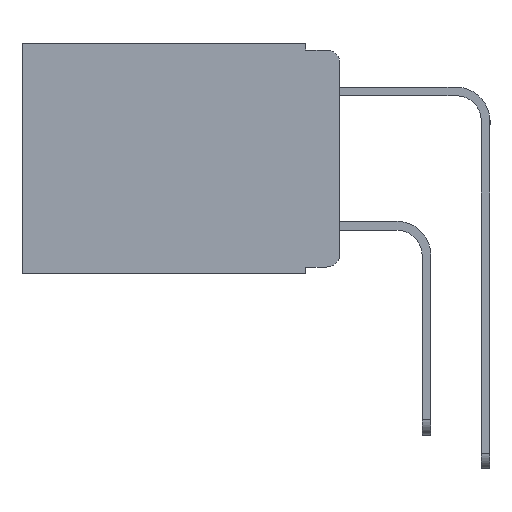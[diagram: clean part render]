
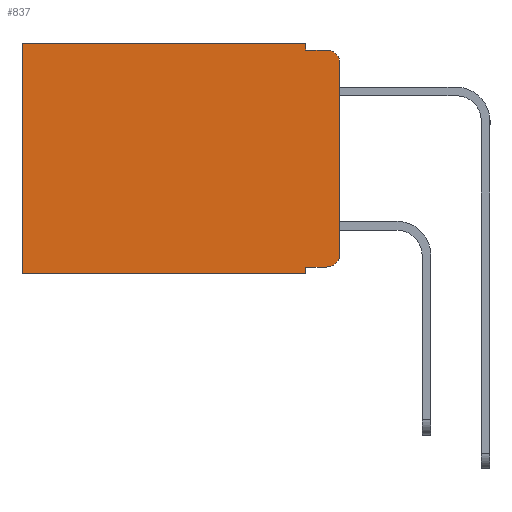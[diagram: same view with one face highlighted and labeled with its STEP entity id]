
A CAD part, left-side view. The second image highlights one B-rep face of the part: STEP entity #837.
In plain terms, the highlighted planar face has unit normal (-1, 0, 0).
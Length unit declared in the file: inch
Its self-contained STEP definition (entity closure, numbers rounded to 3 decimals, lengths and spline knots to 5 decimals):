
#44 = CARTESIAN_POINT ( 'NONE',  ( 0.298, 0., -0.343 ) ) ;
#300 = CIRCLE ( 'NONE', #15026, 0.02 ) ;
#590 = DIRECTION ( 'NONE',  ( 0., 0., -1. ) ) ;
#837 = ADVANCED_FACE ( 'NONE', ( #17397 ), #5609, .F. ) ;
#901 = DIRECTION ( 'NONE',  ( 0., 0., -1. ) ) ;
#1458 = VERTEX_POINT ( 'NONE', #9337 ) ;
#1536 = EDGE_CURVE ( 'NONE', #2580, #4755, #14142, .T. ) ;
#1682 = DIRECTION ( 'NONE',  ( 1., 0., 0. ) ) ;
#1812 = LINE ( 'NONE', #17218, #8643 ) ;
#2066 = CARTESIAN_POINT ( 'NONE',  ( 0.298, 0.473, 0. ) ) ;
#2218 = DIRECTION ( 'NONE',  ( -1., 0., 0. ) ) ;
#2278 = DIRECTION ( 'NONE',  ( 0., -1., 0. ) ) ;
#2351 = VERTEX_POINT ( 'NONE', #14316 ) ;
#2580 = VERTEX_POINT ( 'NONE', #3429 ) ;
#2722 = VECTOR ( 'NONE', #11802, 39.37008 ) ;
#2741 = ORIENTED_EDGE ( 'NONE', *, *, #3618, .F. ) ;
#2819 = CARTESIAN_POINT ( 'NONE',  ( 0.298, 0.051, 0. ) ) ;
#3107 = VECTOR ( 'NONE', #4114, 39.37008 ) ;
#3253 = EDGE_CURVE ( 'NONE', #2351, #4755, #1812, .T. ) ;
#3304 = DIRECTION ( 'NONE',  ( 0., 0., -1. ) ) ;
#3429 = CARTESIAN_POINT ( 'NONE',  ( 0.298, 0.02, -0.333 ) ) ;
#3611 = ORIENTED_EDGE ( 'NONE', *, *, #16328, .F. ) ;
#3618 = EDGE_CURVE ( 'NONE', #8045, #9236, #7158, .T. ) ;
#3931 = VECTOR ( 'NONE', #590, 39.37008 ) ;
#3989 = CARTESIAN_POINT ( 'NONE',  ( 0.298, 0.473, 0. ) ) ;
#4114 = DIRECTION ( 'NONE',  ( 0., 1., 0. ) ) ;
#4152 = AXIS2_PLACEMENT_3D ( 'NONE', #11030, #1682, #10770 ) ;
#4343 = LINE ( 'NONE', #2066, #3931 ) ;
#4755 = VERTEX_POINT ( 'NONE', #6860 ) ;
#4945 = VERTEX_POINT ( 'NONE', #16501 ) ;
#4966 = CARTESIAN_POINT ( 'NONE',  ( 0.298, 0.473, -0.343 ) ) ;
#5494 = ORIENTED_EDGE ( 'NONE', *, *, #7493, .T. ) ;
#5609 = PLANE ( 'NONE',  #4152 ) ;
#5837 = DIRECTION ( 'NONE',  ( -1., 0., 0. ) ) ;
#5928 = ORIENTED_EDGE ( 'NONE', *, *, #15274, .T. ) ;
#6097 = DIRECTION ( 'NONE',  ( 0., 1., 0. ) ) ;
#6785 = ORIENTED_EDGE ( 'NONE', *, *, #3253, .F. ) ;
#6860 = CARTESIAN_POINT ( 'NONE',  ( 0.298, 0., -0.313 ) ) ;
#7158 = LINE ( 'NONE', #44, #3107 ) ;
#7361 = AXIS2_PLACEMENT_3D ( 'NONE', #12222, #5837, #11647 ) ;
#7493 = EDGE_CURVE ( 'NONE', #12480, #13552, #8487, .T. ) ;
#8045 = VERTEX_POINT ( 'NONE', #13812 ) ;
#8256 = EDGE_CURVE ( 'NONE', #2351, #1458, #300, .T. ) ;
#8300 = EDGE_CURVE ( 'NONE', #4945, #2580, #17018, .T. ) ;
#8487 = LINE ( 'NONE', #8618, #15176 ) ;
#8618 = CARTESIAN_POINT ( 'NONE',  ( 0.298, 0., 0. ) ) ;
#8643 = VECTOR ( 'NONE', #17198, 39.37008 ) ;
#8720 = EDGE_CURVE ( 'NONE', #11048, #1458, #13982, .T. ) ;
#9236 = VERTEX_POINT ( 'NONE', #4966 ) ;
#9337 = CARTESIAN_POINT ( 'NONE',  ( 0.298, 0.02, -0.01 ) ) ;
#10429 = VECTOR ( 'NONE', #2278, 39.37008 ) ;
#10770 = DIRECTION ( 'NONE',  ( 0., 0., -1. ) ) ;
#10808 = LINE ( 'NONE', #14158, #16948 ) ;
#10879 = LINE ( 'NONE', #13105, #2722 ) ;
#11030 = CARTESIAN_POINT ( 'NONE',  ( 0.298, 0., 0. ) ) ;
#11048 = VERTEX_POINT ( 'NONE', #15604 ) ;
#11429 = CARTESIAN_POINT ( 'NONE',  ( 0.298, 0.051, -0.01 ) ) ;
#11647 = DIRECTION ( 'NONE',  ( 0., 0., -1. ) ) ;
#11802 = DIRECTION ( 'NONE',  ( 0., 0., -1. ) ) ;
#12164 = ORIENTED_EDGE ( 'NONE', *, *, #8720, .F. ) ;
#12222 = CARTESIAN_POINT ( 'NONE',  ( 0.298, 0.02, -0.313 ) ) ;
#12480 = VERTEX_POINT ( 'NONE', #2819 ) ;
#12805 = EDGE_CURVE ( 'NONE', #12480, #11048, #10879, .T. ) ;
#12919 = CARTESIAN_POINT ( 'NONE',  ( 0.298, 0.02, -0.03 ) ) ;
#13105 = CARTESIAN_POINT ( 'NONE',  ( 0.298, 0.051, 0. ) ) ;
#13552 = VERTEX_POINT ( 'NONE', #3989 ) ;
#13576 = VECTOR ( 'NONE', #15730, 39.37008 ) ;
#13812 = CARTESIAN_POINT ( 'NONE',  ( 0.298, 0.051, -0.343 ) ) ;
#13982 = LINE ( 'NONE', #11429, #10429 ) ;
#14121 = EDGE_LOOP ( 'NONE', ( #6785, #14409, #12164, #15800, #5494, #5928, #2741, #3611, #14423, #16845 ) ) ;
#14142 = CIRCLE ( 'NONE', #7361, 0.02 ) ;
#14158 = CARTESIAN_POINT ( 'NONE',  ( 0.298, 0.051, 0. ) ) ;
#14316 = CARTESIAN_POINT ( 'NONE',  ( 0.298, 0., -0.03 ) ) ;
#14409 = ORIENTED_EDGE ( 'NONE', *, *, #8256, .T. ) ;
#14423 = ORIENTED_EDGE ( 'NONE', *, *, #8300, .T. ) ;
#15026 = AXIS2_PLACEMENT_3D ( 'NONE', #12919, #2218, #901 ) ;
#15176 = VECTOR ( 'NONE', #6097, 39.37008 ) ;
#15274 = EDGE_CURVE ( 'NONE', #13552, #9236, #4343, .T. ) ;
#15604 = CARTESIAN_POINT ( 'NONE',  ( 0.298, 0.051, -0.01 ) ) ;
#15730 = DIRECTION ( 'NONE',  ( 0., -1., 0. ) ) ;
#15800 = ORIENTED_EDGE ( 'NONE', *, *, #12805, .F. ) ;
#15877 = CARTESIAN_POINT ( 'NONE',  ( 0.298, 0.051, -0.333 ) ) ;
#16328 = EDGE_CURVE ( 'NONE', #4945, #8045, #10808, .T. ) ;
#16501 = CARTESIAN_POINT ( 'NONE',  ( 0.298, 0.051, -0.333 ) ) ;
#16845 = ORIENTED_EDGE ( 'NONE', *, *, #1536, .T. ) ;
#16948 = VECTOR ( 'NONE', #3304, 39.37008 ) ;
#17018 = LINE ( 'NONE', #15877, #13576 ) ;
#17198 = DIRECTION ( 'NONE',  ( 0., 0., -1. ) ) ;
#17218 = CARTESIAN_POINT ( 'NONE',  ( 0.298, 0., 0. ) ) ;
#17397 = FACE_OUTER_BOUND ( 'NONE', #14121, .T. ) ;
